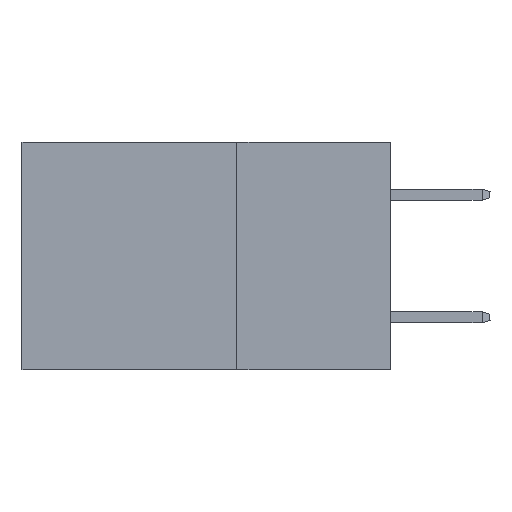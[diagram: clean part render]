
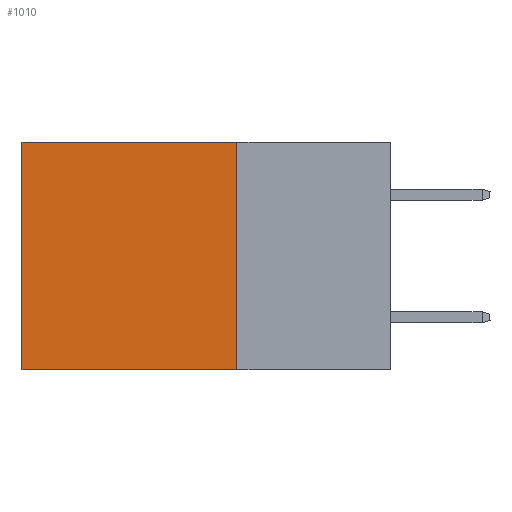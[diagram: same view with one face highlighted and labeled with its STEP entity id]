
A CAD part, left-side view. The second image highlights one B-rep face of the part: STEP entity #1010.
In plain terms, the highlighted planar face has unit normal (-1, 0, 0).
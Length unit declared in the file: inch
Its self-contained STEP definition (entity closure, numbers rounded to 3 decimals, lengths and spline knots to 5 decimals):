
#72 = LINE ( 'NONE', #1862, #9463 ) ;
#398 = DIRECTION ( 'NONE',  ( 0., 0., -1. ) ) ;
#645 = DIRECTION ( 'NONE',  ( 0., 1., 0. ) ) ;
#707 = CARTESIAN_POINT ( 'NONE',  ( 0.2875, 0.25, 0. ) ) ;
#929 = VERTEX_POINT ( 'NONE', #8416 ) ;
#1010 = ADVANCED_FACE ( 'NONE', ( #9881 ), #2055, .F. ) ;
#1477 = DIRECTION ( 'NONE',  ( 0., 0., -1. ) ) ;
#1509 = VERTEX_POINT ( 'NONE', #10947 ) ;
#1809 = VECTOR ( 'NONE', #5299, 39.37008 ) ;
#1862 = CARTESIAN_POINT ( 'NONE',  ( 0.2875, 0.6, 0. ) ) ;
#1893 = EDGE_CURVE ( 'NONE', #9705, #5903, #3310, .T. ) ;
#2017 = VECTOR ( 'NONE', #645, 39.37008 ) ;
#2055 = PLANE ( 'NONE',  #9421 ) ;
#2184 = EDGE_CURVE ( 'NONE', #1509, #929, #72, .T. ) ;
#2242 = EDGE_CURVE ( 'NONE', #9705, #1509, #6859, .T. ) ;
#3310 = LINE ( 'NONE', #4244, #10126 ) ;
#3604 = ORIENTED_EDGE ( 'NONE', *, *, #2184, .T. ) ;
#3895 = ORIENTED_EDGE ( 'NONE', *, *, #4007, .F. ) ;
#4007 = EDGE_CURVE ( 'NONE', #5903, #929, #8727, .T. ) ;
#4244 = CARTESIAN_POINT ( 'NONE',  ( 0.2875, 0.25, 0. ) ) ;
#4262 = DIRECTION ( 'NONE',  ( 0., 0., -1. ) ) ;
#4290 = ORIENTED_EDGE ( 'NONE', *, *, #1893, .F. ) ;
#5044 = ORIENTED_EDGE ( 'NONE', *, *, #2242, .T. ) ;
#5294 = CARTESIAN_POINT ( 'NONE',  ( 0.2875, 0.25, -0.37 ) ) ;
#5299 = DIRECTION ( 'NONE',  ( 0., 1., 0. ) ) ;
#5903 = VERTEX_POINT ( 'NONE', #7146 ) ;
#6751 = EDGE_LOOP ( 'NONE', ( #3604, #3895, #4290, #5044 ) ) ;
#6859 = LINE ( 'NONE', #707, #2017 ) ;
#7119 = CARTESIAN_POINT ( 'NONE',  ( 0.2875, 0.25, 0. ) ) ;
#7146 = CARTESIAN_POINT ( 'NONE',  ( 0.2875, 0.25, -0.37 ) ) ;
#7670 = CARTESIAN_POINT ( 'NONE',  ( 0.2875, 0.25, 0. ) ) ;
#8416 = CARTESIAN_POINT ( 'NONE',  ( 0.2875, 0.6, -0.37 ) ) ;
#8727 = LINE ( 'NONE', #5294, #1809 ) ;
#9421 = AXIS2_PLACEMENT_3D ( 'NONE', #7119, #10047, #398 ) ;
#9463 = VECTOR ( 'NONE', #1477, 39.37008 ) ;
#9705 = VERTEX_POINT ( 'NONE', #7670 ) ;
#9881 = FACE_OUTER_BOUND ( 'NONE', #6751, .T. ) ;
#10047 = DIRECTION ( 'NONE',  ( 1., 0., 0. ) ) ;
#10126 = VECTOR ( 'NONE', #4262, 39.37008 ) ;
#10947 = CARTESIAN_POINT ( 'NONE',  ( 0.2875, 0.6, 0. ) ) ;
